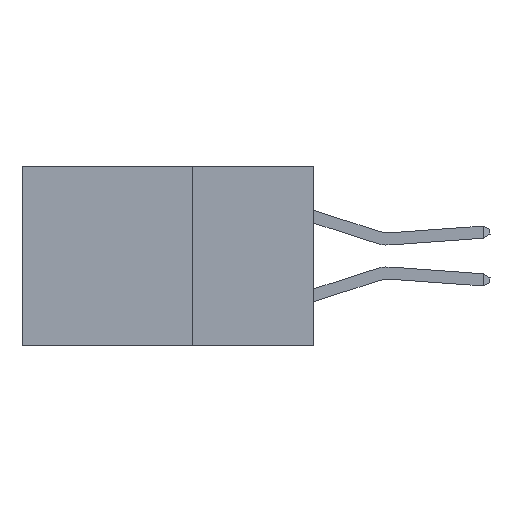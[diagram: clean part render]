
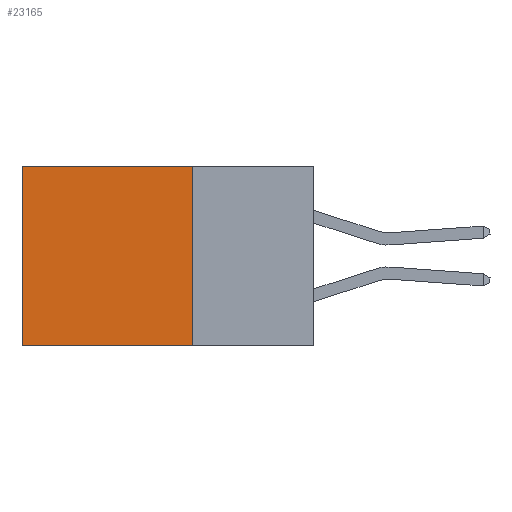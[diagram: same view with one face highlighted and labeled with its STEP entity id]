
A CAD part, left-side view. The second image highlights one B-rep face of the part: STEP entity #23165.
In plain terms, the highlighted planar face has unit normal (-1, 0, 0).
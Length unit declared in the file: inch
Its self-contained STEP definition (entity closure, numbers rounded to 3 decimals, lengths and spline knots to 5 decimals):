
#801 = CARTESIAN_POINT ( 'NONE',  ( 0.2875, 0.25, 0. ) ) ;
#997 = ORIENTED_EDGE ( 'NONE', *, *, #14620, .F. ) ;
#1859 = DIRECTION ( 'NONE',  ( 0., 0., -1. ) ) ;
#2502 = VECTOR ( 'NONE', #19551, 39.37008 ) ;
#4293 = DIRECTION ( 'NONE',  ( 0., 0., -1. ) ) ;
#4487 = VERTEX_POINT ( 'NONE', #11733 ) ;
#6530 = ORIENTED_EDGE ( 'NONE', *, *, #20762, .T. ) ;
#6683 = VECTOR ( 'NONE', #21656, 39.37008 ) ;
#8524 = ORIENTED_EDGE ( 'NONE', *, *, #14705, .F. ) ;
#8572 = LINE ( 'NONE', #801, #6683 ) ;
#10222 = LINE ( 'NONE', #37985, #17301 ) ;
#10510 = CARTESIAN_POINT ( 'NONE',  ( 0.2875, 0.25, 0. ) ) ;
#11252 = VERTEX_POINT ( 'NONE', #12255 ) ;
#11620 = VERTEX_POINT ( 'NONE', #10510 ) ;
#11733 = CARTESIAN_POINT ( 'NONE',  ( 0.2875, 0.6, -0.37 ) ) ;
#12255 = CARTESIAN_POINT ( 'NONE',  ( 0.2875, 0.25, -0.37 ) ) ;
#13010 = AXIS2_PLACEMENT_3D ( 'NONE', #37143, #31635, #4293 ) ;
#14620 = EDGE_CURVE ( 'NONE', #11620, #11252, #8572, .T. ) ;
#14705 = EDGE_CURVE ( 'NONE', #11252, #4487, #19835, .T. ) ;
#16463 = VERTEX_POINT ( 'NONE', #33336 ) ;
#16972 = EDGE_CURVE ( 'NONE', #11620, #16463, #10222, .T. ) ;
#17301 = VECTOR ( 'NONE', #22849, 39.37008 ) ;
#19551 = DIRECTION ( 'NONE',  ( 0., 1., 0. ) ) ;
#19718 = VECTOR ( 'NONE', #1859, 39.37008 ) ;
#19835 = LINE ( 'NONE', #31413, #2502 ) ;
#20762 = EDGE_CURVE ( 'NONE', #16463, #4487, #26769, .T. ) ;
#21656 = DIRECTION ( 'NONE',  ( 0., 0., -1. ) ) ;
#22849 = DIRECTION ( 'NONE',  ( 0., 1., 0. ) ) ;
#22963 = CARTESIAN_POINT ( 'NONE',  ( 0.2875, 0.6, 0. ) ) ;
#23165 = ADVANCED_FACE ( 'NONE', ( #23261 ), #34631, .F. ) ;
#23261 = FACE_OUTER_BOUND ( 'NONE', #34645, .T. ) ;
#26769 = LINE ( 'NONE', #22963, #19718 ) ;
#31413 = CARTESIAN_POINT ( 'NONE',  ( 0.2875, 0.25, -0.37 ) ) ;
#31635 = DIRECTION ( 'NONE',  ( 1., 0., 0. ) ) ;
#33336 = CARTESIAN_POINT ( 'NONE',  ( 0.2875, 0.6, 0. ) ) ;
#34631 = PLANE ( 'NONE',  #13010 ) ;
#34645 = EDGE_LOOP ( 'NONE', ( #6530, #8524, #997, #35771 ) ) ;
#35771 = ORIENTED_EDGE ( 'NONE', *, *, #16972, .T. ) ;
#37143 = CARTESIAN_POINT ( 'NONE',  ( 0.2875, 0.25, 0. ) ) ;
#37985 = CARTESIAN_POINT ( 'NONE',  ( 0.2875, 0.25, 0. ) ) ;
